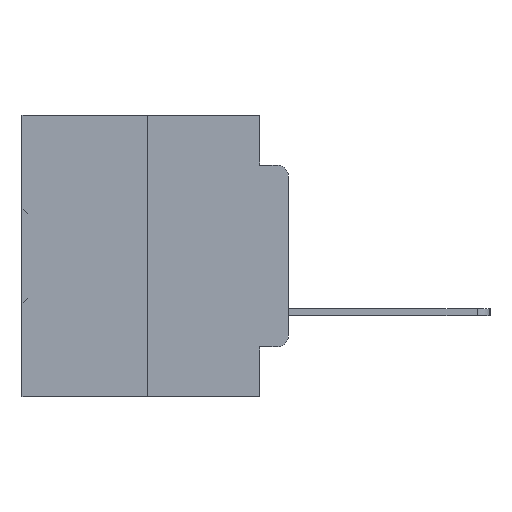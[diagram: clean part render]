
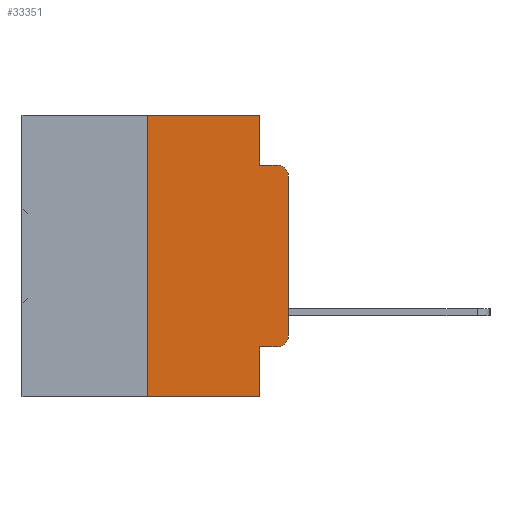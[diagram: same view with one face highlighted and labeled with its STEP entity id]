
A CAD part, left-side view. The second image highlights one B-rep face of the part: STEP entity #33351.
In plain terms, the highlighted planar face has unit normal (-1, 0, 0).
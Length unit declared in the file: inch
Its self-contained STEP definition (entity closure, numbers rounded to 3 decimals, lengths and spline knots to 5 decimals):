
#590 = VECTOR ( 'NONE', #15405, 39.37008 ) ;
#910 = VECTOR ( 'NONE', #27372, 39.37008 ) ;
#1417 = ORIENTED_EDGE ( 'NONE', *, *, #16928, .T. ) ;
#1487 = DIRECTION ( 'NONE',  ( 0., 0., -1. ) ) ;
#1755 = PLANE ( 'NONE',  #6961 ) ;
#1770 = CARTESIAN_POINT ( 'NONE',  ( 0., 0.473, 0. ) ) ;
#2309 = EDGE_CURVE ( 'NONE', #14452, #14119, #25554, .T. ) ;
#2562 = CARTESIAN_POINT ( 'NONE',  ( 0., 0.02, -0.3915 ) ) ;
#3226 = VERTEX_POINT ( 'NONE', #18882 ) ;
#3324 = EDGE_CURVE ( 'NONE', #21635, #3226, #14560, .T. ) ;
#3759 = ORIENTED_EDGE ( 'NONE', *, *, #24680, .T. ) ;
#4786 = EDGE_CURVE ( 'NONE', #14119, #29228, #14489, .T. ) ;
#4805 = CARTESIAN_POINT ( 'NONE',  ( 0., 0., -0.1085 ) ) ;
#5610 = LINE ( 'NONE', #1770, #34416 ) ;
#5705 = DIRECTION ( 'NONE',  ( -1., 0., 0. ) ) ;
#5728 = CARTESIAN_POINT ( 'NONE',  ( 0., 0., -0.3915 ) ) ;
#6027 = VERTEX_POINT ( 'NONE', #21181 ) ;
#6961 = AXIS2_PLACEMENT_3D ( 'NONE', #21442, #7418, #27048 ) ;
#6962 = VECTOR ( 'NONE', #17915, 39.37008 ) ;
#7206 = EDGE_CURVE ( 'NONE', #30160, #14452, #20125, .T. ) ;
#7418 = DIRECTION ( 'NONE',  ( 1., 0., 0. ) ) ;
#7746 = CARTESIAN_POINT ( 'NONE',  ( 0., 0.051, 0. ) ) ;
#7849 = EDGE_CURVE ( 'NONE', #30160, #18064, #28770, .T. ) ;
#8389 = LINE ( 'NONE', #7746, #910 ) ;
#8687 = AXIS2_PLACEMENT_3D ( 'NONE', #22551, #5705, #25338 ) ;
#9067 = CARTESIAN_POINT ( 'NONE',  ( 0., 0.25, -0.5 ) ) ;
#10029 = CARTESIAN_POINT ( 'NONE',  ( 0., 0.051, -0.4115 ) ) ;
#10448 = DIRECTION ( 'NONE',  ( 0., -1., 0. ) ) ;
#11722 = VECTOR ( 'NONE', #12896, 39.37008 ) ;
#12862 = CARTESIAN_POINT ( 'NONE',  ( 0., 0.02, -0.4115 ) ) ;
#12896 = DIRECTION ( 'NONE',  ( 0., -1., 0. ) ) ;
#13032 = VECTOR ( 'NONE', #1487, 39.37008 ) ;
#14119 = VERTEX_POINT ( 'NONE', #5728 ) ;
#14452 = VERTEX_POINT ( 'NONE', #12862 ) ;
#14489 = LINE ( 'NONE', #28880, #6962 ) ;
#14560 = LINE ( 'NONE', #33037, #28544 ) ;
#15405 = DIRECTION ( 'NONE',  ( 0., -1., 0. ) ) ;
#16438 = DIRECTION ( 'NONE',  ( 0., 0., 1. ) ) ;
#16928 = EDGE_CURVE ( 'NONE', #29228, #33469, #34820, .T. ) ;
#16929 = ORIENTED_EDGE ( 'NONE', *, *, #27737, .F. ) ;
#17915 = DIRECTION ( 'NONE',  ( 0., 0., 1. ) ) ;
#18064 = VERTEX_POINT ( 'NONE', #27453 ) ;
#18674 = DIRECTION ( 'NONE',  ( 0., -1., 0. ) ) ;
#18882 = CARTESIAN_POINT ( 'NONE',  ( 0., 0.25, 0. ) ) ;
#19994 = ORIENTED_EDGE ( 'NONE', *, *, #3324, .F. ) ;
#20125 = LINE ( 'NONE', #10029, #11722 ) ;
#21181 = CARTESIAN_POINT ( 'NONE',  ( 0., 0.051, -0.0885 ) ) ;
#21442 = CARTESIAN_POINT ( 'NONE',  ( 0., 0.473, 0. ) ) ;
#21635 = VERTEX_POINT ( 'NONE', #9067 ) ;
#21927 = DIRECTION ( 'NONE',  ( -1., 0., 0. ) ) ;
#22551 = CARTESIAN_POINT ( 'NONE',  ( 0., 0.02, -0.1085 ) ) ;
#22708 = VECTOR ( 'NONE', #10448, 39.37008 ) ;
#23247 = EDGE_CURVE ( 'NONE', #6027, #33469, #30402, .T. ) ;
#23367 = CARTESIAN_POINT ( 'NONE',  ( 0., 0.051, 0. ) ) ;
#23581 = LINE ( 'NONE', #24450, #22708 ) ;
#24450 = CARTESIAN_POINT ( 'NONE',  ( 0., 0.473, -0.5 ) ) ;
#24680 = EDGE_CURVE ( 'NONE', #21635, #18064, #23581, .T. ) ;
#25338 = DIRECTION ( 'NONE',  ( 0., 0., -1. ) ) ;
#25542 = ORIENTED_EDGE ( 'NONE', *, *, #7849, .F. ) ;
#25554 = CIRCLE ( 'NONE', #29319, 0.02 ) ;
#25740 = CARTESIAN_POINT ( 'NONE',  ( 0., 0.051, -0.4115 ) ) ;
#26913 = ORIENTED_EDGE ( 'NONE', *, *, #2309, .T. ) ;
#27048 = DIRECTION ( 'NONE',  ( 0., 0., -1. ) ) ;
#27372 = DIRECTION ( 'NONE',  ( 0., 0., -1. ) ) ;
#27453 = CARTESIAN_POINT ( 'NONE',  ( 0., 0.051, -0.5 ) ) ;
#27475 = VERTEX_POINT ( 'NONE', #23367 ) ;
#27529 = CARTESIAN_POINT ( 'NONE',  ( 0., 0.02, -0.0885 ) ) ;
#27737 = EDGE_CURVE ( 'NONE', #27475, #6027, #8389, .T. ) ;
#28544 = VECTOR ( 'NONE', #16438, 39.37008 ) ;
#28770 = LINE ( 'NONE', #32205, #13032 ) ;
#28880 = CARTESIAN_POINT ( 'NONE',  ( 0., 0., 0. ) ) ;
#29228 = VERTEX_POINT ( 'NONE', #4805 ) ;
#29299 = CARTESIAN_POINT ( 'NONE',  ( 0., 0.051, -0.0885 ) ) ;
#29319 = AXIS2_PLACEMENT_3D ( 'NONE', #2562, #21927, #32519 ) ;
#30129 = FACE_OUTER_BOUND ( 'NONE', #30392, .T. ) ;
#30160 = VERTEX_POINT ( 'NONE', #25740 ) ;
#30392 = EDGE_LOOP ( 'NONE', ( #30777, #1417, #32937, #16929, #33394, #19994, #3759, #25542, #34619, #26913 ) ) ;
#30402 = LINE ( 'NONE', #29299, #590 ) ;
#30777 = ORIENTED_EDGE ( 'NONE', *, *, #4786, .T. ) ;
#32205 = CARTESIAN_POINT ( 'NONE',  ( 0., 0.051, 0. ) ) ;
#32519 = DIRECTION ( 'NONE',  ( 0., 0., -1. ) ) ;
#32937 = ORIENTED_EDGE ( 'NONE', *, *, #23247, .F. ) ;
#33037 = CARTESIAN_POINT ( 'NONE',  ( 0., 0.25, 0. ) ) ;
#33351 = ADVANCED_FACE ( 'NONE', ( #30129 ), #1755, .F. ) ;
#33394 = ORIENTED_EDGE ( 'NONE', *, *, #35113, .F. ) ;
#33469 = VERTEX_POINT ( 'NONE', #27529 ) ;
#34416 = VECTOR ( 'NONE', #18674, 39.37008 ) ;
#34619 = ORIENTED_EDGE ( 'NONE', *, *, #7206, .T. ) ;
#34820 = CIRCLE ( 'NONE', #8687, 0.02 ) ;
#35113 = EDGE_CURVE ( 'NONE', #3226, #27475, #5610, .T. ) ;
